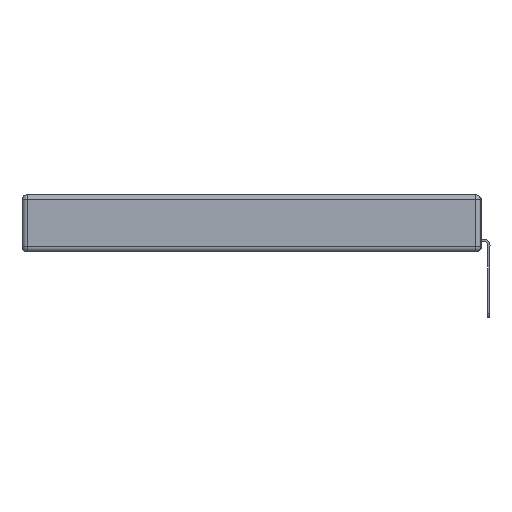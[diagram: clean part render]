
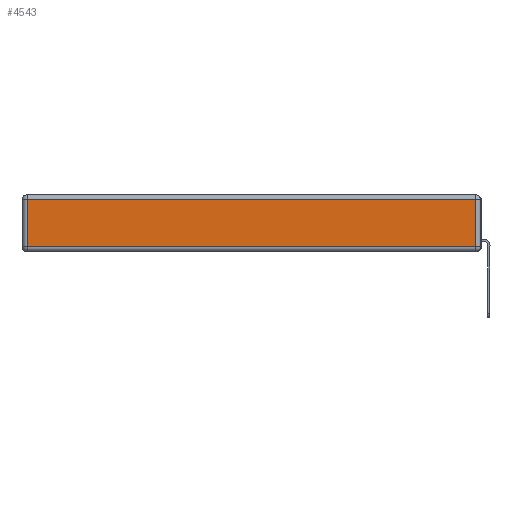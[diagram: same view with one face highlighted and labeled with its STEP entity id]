
A CAD part, left-side view. The second image highlights one B-rep face of the part: STEP entity #4543.
In plain terms, the highlighted planar face has unit normal (-1, 0, 0).
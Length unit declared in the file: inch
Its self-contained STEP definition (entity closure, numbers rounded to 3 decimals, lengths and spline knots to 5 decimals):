
#1061 = CARTESIAN_POINT ( 'NONE',  ( 0., 0.03, -0.03 ) ) ;
#2431 = EDGE_CURVE ( 'NONE', #8522, #12873, #18476, .T. ) ;
#4469 = EDGE_CURVE ( 'NONE', #17286, #8522, #17377, .T. ) ;
#4543 = ADVANCED_FACE ( 'NONE', ( #17015 ), #24857, .T. ) ;
#4849 = CARTESIAN_POINT ( 'NONE',  ( 0., 0.03, -0.343 ) ) ;
#5755 = CARTESIAN_POINT ( 'NONE',  ( 0., 2.72, -0.313 ) ) ;
#5790 = VECTOR ( 'NONE', #12015, 39.37008 ) ;
#8493 = ORIENTED_EDGE ( 'NONE', *, *, #15257, .T. ) ;
#8522 = VERTEX_POINT ( 'NONE', #5755 ) ;
#11653 = VECTOR ( 'NONE', #18864, 39.37008 ) ;
#12015 = DIRECTION ( 'NONE',  ( 0., 0., 1. ) ) ;
#12624 = EDGE_CURVE ( 'NONE', #12873, #23162, #14867, .T. ) ;
#12873 = VERTEX_POINT ( 'NONE', #27743 ) ;
#13043 = CARTESIAN_POINT ( 'NONE',  ( 0., 2.72, -0.03 ) ) ;
#13114 = ORIENTED_EDGE ( 'NONE', *, *, #12624, .T. ) ;
#13717 = CARTESIAN_POINT ( 'NONE',  ( 0., 0., -0.313 ) ) ;
#14198 = DIRECTION ( 'NONE',  ( -1., 0., 0. ) ) ;
#14867 = LINE ( 'NONE', #4849, #5790 ) ;
#15174 = EDGE_LOOP ( 'NONE', ( #18374, #13114, #8493, #20921 ) ) ;
#15257 = EDGE_CURVE ( 'NONE', #23162, #17286, #24210, .T. ) ;
#15458 = AXIS2_PLACEMENT_3D ( 'NONE', #22526, #14198, #26717 ) ;
#15857 = DIRECTION ( 'NONE',  ( 0., -1., 0. ) ) ;
#16411 = VECTOR ( 'NONE', #18147, 39.37008 ) ;
#16427 = VECTOR ( 'NONE', #15857, 39.37008 ) ;
#16590 = CARTESIAN_POINT ( 'NONE',  ( 0., 2.72, -0.343 ) ) ;
#17015 = FACE_OUTER_BOUND ( 'NONE', #15174, .T. ) ;
#17286 = VERTEX_POINT ( 'NONE', #13043 ) ;
#17377 = LINE ( 'NONE', #16590, #11653 ) ;
#18147 = DIRECTION ( 'NONE',  ( 0., 1., 0. ) ) ;
#18374 = ORIENTED_EDGE ( 'NONE', *, *, #2431, .T. ) ;
#18476 = LINE ( 'NONE', #13717, #16427 ) ;
#18864 = DIRECTION ( 'NONE',  ( 0., 0., -1. ) ) ;
#20921 = ORIENTED_EDGE ( 'NONE', *, *, #4469, .T. ) ;
#22526 = CARTESIAN_POINT ( 'NONE',  ( 0., 0., -0.343 ) ) ;
#23162 = VERTEX_POINT ( 'NONE', #1061 ) ;
#24210 = LINE ( 'NONE', #26723, #16411 ) ;
#24857 = PLANE ( 'NONE',  #15458 ) ;
#26717 = DIRECTION ( 'NONE',  ( 0., 0., 1. ) ) ;
#26723 = CARTESIAN_POINT ( 'NONE',  ( 0., 2.75, -0.03 ) ) ;
#27743 = CARTESIAN_POINT ( 'NONE',  ( 0., 0.03, -0.313 ) ) ;
